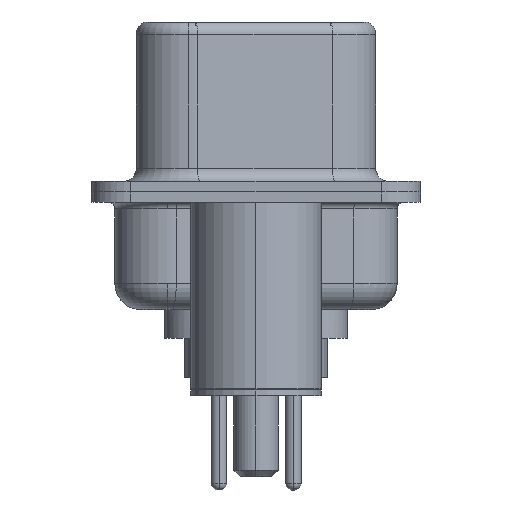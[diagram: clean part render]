
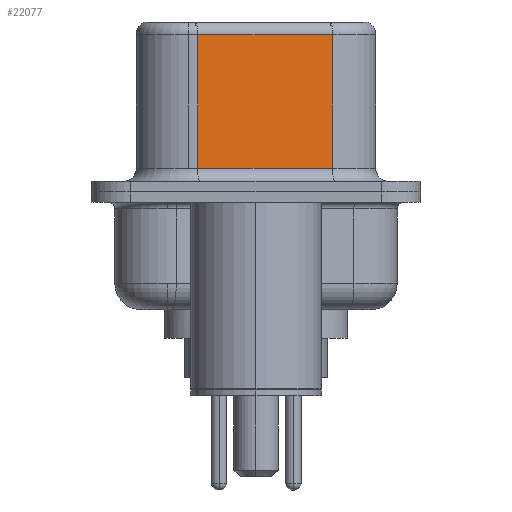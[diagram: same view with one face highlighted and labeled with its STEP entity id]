
A CAD part, left-side view. The second image highlights one B-rep face of the part: STEP entity #22077.
In plain terms, the highlighted planar face has unit normal (-0.985, -0.174, 0).
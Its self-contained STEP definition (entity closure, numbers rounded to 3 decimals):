
#67 = VERTEX_POINT ( 'NONE', #4534 ) ;
#1073 = CARTESIAN_POINT ( 'NONE',  ( 3.67, 2.233, 6.52 ) ) ;
#1160 = LINE ( 'NONE', #9967, #20290 ) ;
#2555 = CARTESIAN_POINT ( 'NONE',  ( 4.58, -2.927, 0.9 ) ) ;
#2708 = VERTEX_POINT ( 'NONE', #23061 ) ;
#3417 = EDGE_CURVE ( 'NONE', #67, #21392, #9167, .T. ) ;
#3915 = EDGE_CURVE ( 'NONE', #2708, #67, #13432, .T. ) ;
#4060 = AXIS2_PLACEMENT_3D ( 'NONE', #8363, #21257, #10271 ) ;
#4196 = VECTOR ( 'NONE', #17428, 1000. ) ;
#4534 = CARTESIAN_POINT ( 'NONE',  ( 3.67, 2.233, 0.9 ) ) ;
#5466 = EDGE_CURVE ( 'NONE', #19771, #2708, #1160, .T. ) ;
#5692 = DIRECTION ( 'NONE',  ( 0., 0., -1. ) ) ;
#7078 = ORIENTED_EDGE ( 'NONE', *, *, #15039, .F. ) ;
#7522 = LINE ( 'NONE', #22632, #16801 ) ;
#7967 = VECTOR ( 'NONE', #5692, 1000. ) ;
#8363 = CARTESIAN_POINT ( 'NONE',  ( 4.58, -2.927, 6.52 ) ) ;
#9167 = LINE ( 'NONE', #2555, #4196 ) ;
#9967 = CARTESIAN_POINT ( 'NONE',  ( 4.58, -2.927, 6.02 ) ) ;
#10271 = DIRECTION ( 'NONE',  ( -0.174, 0.985, 0. ) ) ;
#11708 = DIRECTION ( 'NONE',  ( 0., 0., -1. ) ) ;
#12008 = CARTESIAN_POINT ( 'NONE',  ( 4.58, -2.927, 0.9 ) ) ;
#12726 = ORIENTED_EDGE ( 'NONE', *, *, #3915, .T. ) ;
#13432 = LINE ( 'NONE', #1073, #7967 ) ;
#15039 = EDGE_CURVE ( 'NONE', #19771, #21392, #7522, .T. ) ;
#16801 = VECTOR ( 'NONE', #11708, 1000. ) ;
#17428 = DIRECTION ( 'NONE',  ( 0.174, -0.985, 0. ) ) ;
#17575 = PLANE ( 'NONE',  #4060 ) ;
#18967 = FACE_OUTER_BOUND ( 'NONE', #20603, .T. ) ;
#19771 = VERTEX_POINT ( 'NONE', #22920 ) ;
#20290 = VECTOR ( 'NONE', #23741, 1000. ) ;
#20603 = EDGE_LOOP ( 'NONE', ( #7078, #20823, #12726, #22428 ) ) ;
#20823 = ORIENTED_EDGE ( 'NONE', *, *, #5466, .T. ) ;
#21257 = DIRECTION ( 'NONE',  ( 0.985, 0.174, 0. ) ) ;
#21392 = VERTEX_POINT ( 'NONE', #12008 ) ;
#22077 = ADVANCED_FACE ( 'NONE', ( #18967 ), #17575, .F. ) ;
#22428 = ORIENTED_EDGE ( 'NONE', *, *, #3417, .T. ) ;
#22632 = CARTESIAN_POINT ( 'NONE',  ( 4.58, -2.927, 6.52 ) ) ;
#22920 = CARTESIAN_POINT ( 'NONE',  ( 4.58, -2.927, 6.02 ) ) ;
#23061 = CARTESIAN_POINT ( 'NONE',  ( 3.67, 2.233, 6.02 ) ) ;
#23741 = DIRECTION ( 'NONE',  ( -0.174, 0.985, 0. ) ) ;
